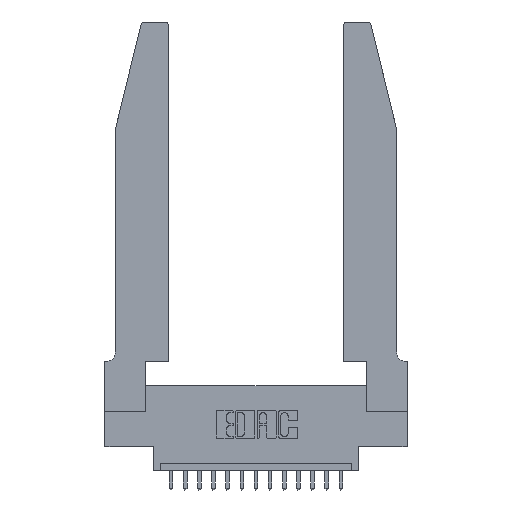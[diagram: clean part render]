
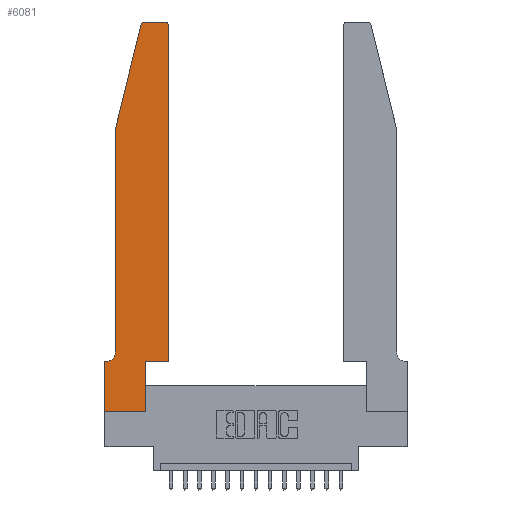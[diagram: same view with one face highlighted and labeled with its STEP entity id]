
A CAD part, top view. The second image highlights one B-rep face of the part: STEP entity #6081.
In plain terms, the highlighted planar face has unit normal (0, 0, 1).
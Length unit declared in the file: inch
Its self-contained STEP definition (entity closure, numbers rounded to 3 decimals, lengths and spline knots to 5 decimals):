
#275 = EDGE_CURVE ( 'NONE', #992, #12603, #14734, .T. ) ;
#431 = ORIENTED_EDGE ( 'NONE', *, *, #1034, .T. ) ;
#802 = LINE ( 'NONE', #11747, #1932 ) ;
#893 = ORIENTED_EDGE ( 'NONE', *, *, #7405, .T. ) ;
#992 = VERTEX_POINT ( 'NONE', #16930 ) ;
#1011 = DIRECTION ( 'NONE',  ( 1., 0., 0. ) ) ;
#1034 = EDGE_CURVE ( 'NONE', #15784, #10803, #11558, .T. ) ;
#1245 = LINE ( 'NONE', #11678, #12207 ) ;
#1253 = ORIENTED_EDGE ( 'NONE', *, *, #7828, .T. ) ;
#1406 = VECTOR ( 'NONE', #17836, 39.37008 ) ;
#1714 = VECTOR ( 'NONE', #6946, 39.37008 ) ;
#1932 = VECTOR ( 'NONE', #6489, 39.37008 ) ;
#2142 = CARTESIAN_POINT ( 'NONE',  ( 0.0755, 0.42, 0.37 ) ) ;
#2252 = ORIENTED_EDGE ( 'NONE', *, *, #5869, .T. ) ;
#2297 = ORIENTED_EDGE ( 'NONE', *, *, #18383, .T. ) ;
#2331 = EDGE_CURVE ( 'NONE', #3110, #8084, #14193, .T. ) ;
#2360 = CARTESIAN_POINT ( 'NONE',  ( 0.4505, 0.35, 0.37 ) ) ;
#2368 = LINE ( 'NONE', #11858, #17186 ) ;
#2920 = CARTESIAN_POINT ( 'NONE',  ( 0.4505, 0.35, 0.37 ) ) ;
#2996 = VECTOR ( 'NONE', #14667, 39.37008 ) ;
#3092 = EDGE_CURVE ( 'NONE', #12421, #7818, #16672, .T. ) ;
#3110 = VERTEX_POINT ( 'NONE', #2142 ) ;
#3122 = CARTESIAN_POINT ( 'NONE',  ( 0.25487, 2.72718, 0.37 ) ) ;
#3151 = DIRECTION ( 'NONE',  ( 0., -1., 0. ) ) ;
#3358 = ORIENTED_EDGE ( 'NONE', *, *, #275, .T. ) ;
#4008 = CARTESIAN_POINT ( 'NONE',  ( 0.284, 2.75, 0.37 ) ) ;
#4767 = CARTESIAN_POINT ( 'NONE',  ( 0.2865, 0., 0.37 ) ) ;
#4780 = CARTESIAN_POINT ( 'NONE',  ( 0.2605, 2.75, 0.37 ) ) ;
#5009 = CARTESIAN_POINT ( 'NONE',  ( 0.4205, 2.75, 0.37 ) ) ;
#5579 = CARTESIAN_POINT ( 'NONE',  ( 0.4505, 2.72, 0.37 ) ) ;
#5681 = LINE ( 'NONE', #9490, #6774 ) ;
#5869 = EDGE_CURVE ( 'NONE', #12247, #12972, #1245, .T. ) ;
#6023 = CARTESIAN_POINT ( 'NONE',  ( 0.4505, 0.35, 0.37 ) ) ;
#6081 = ADVANCED_FACE ( 'NONE', ( #13784 ), #17409, .T. ) ;
#6287 = EDGE_CURVE ( 'NONE', #8084, #18220, #2368, .T. ) ;
#6299 = EDGE_CURVE ( 'NONE', #10803, #992, #802, .T. ) ;
#6489 = DIRECTION ( 'NONE',  ( 0., 1., 0. ) ) ;
#6620 = ORIENTED_EDGE ( 'NONE', *, *, #6299, .T. ) ;
#6774 = VECTOR ( 'NONE', #18067, 39.37008 ) ;
#6930 = ORIENTED_EDGE ( 'NONE', *, *, #15276, .T. ) ;
#6946 = DIRECTION ( 'NONE',  ( 1., 0., 0. ) ) ;
#7000 = DIRECTION ( 'NONE',  ( 0., 0., 1. ) ) ;
#7405 = EDGE_CURVE ( 'NONE', #12603, #15984, #17155, .T. ) ;
#7805 = CARTESIAN_POINT ( 'NONE',  ( 0., 0.35, 0.37 ) ) ;
#7818 = VERTEX_POINT ( 'NONE', #4008 ) ;
#7828 = EDGE_CURVE ( 'NONE', #7818, #12247, #18034, .T. ) ;
#8000 = VECTOR ( 'NONE', #12932, 39.37008 ) ;
#8084 = VERTEX_POINT ( 'NONE', #15748 ) ;
#8209 = AXIS2_PLACEMENT_3D ( 'NONE', #16126, #17591, #13353 ) ;
#8417 = CIRCLE ( 'NONE', #18144, 0.03 ) ;
#8567 = ORIENTED_EDGE ( 'NONE', *, *, #3092, .T. ) ;
#8628 = ORIENTED_EDGE ( 'NONE', *, *, #6287, .T. ) ;
#8824 = CARTESIAN_POINT ( 'NONE',  ( 0.0755, 2., 0.37 ) ) ;
#8908 = DIRECTION ( 'NONE',  ( 0., 0., 1. ) ) ;
#9490 = CARTESIAN_POINT ( 'NONE',  ( 0., 0., 0.37 ) ) ;
#9697 = AXIS2_PLACEMENT_3D ( 'NONE', #13235, #8908, #16075 ) ;
#10175 = ORIENTED_EDGE ( 'NONE', *, *, #11659, .T. ) ;
#10605 = CARTESIAN_POINT ( 'NONE',  ( 0.0755, 2., 0.37 ) ) ;
#10803 = VERTEX_POINT ( 'NONE', #4767 ) ;
#10915 = ORIENTED_EDGE ( 'NONE', *, *, #2331, .T. ) ;
#11319 = DIRECTION ( 'NONE',  ( 1., 0., 0. ) ) ;
#11504 = DIRECTION ( 'NONE',  ( -0.239, -0.971, 0. ) ) ;
#11558 = LINE ( 'NONE', #14008, #1714 ) ;
#11659 = EDGE_CURVE ( 'NONE', #12972, #3110, #17326, .T. ) ;
#11678 = CARTESIAN_POINT ( 'NONE',  ( 0.0755, 2., 0.37 ) ) ;
#11747 = CARTESIAN_POINT ( 'NONE',  ( 0.2865, 0.35, 0.37 ) ) ;
#11858 = CARTESIAN_POINT ( 'NONE',  ( 0.0755, 0.35, 0.37 ) ) ;
#12121 = VECTOR ( 'NONE', #3151, 39.37008 ) ;
#12207 = VECTOR ( 'NONE', #11504, 39.37008 ) ;
#12247 = VERTEX_POINT ( 'NONE', #3122 ) ;
#12421 = VERTEX_POINT ( 'NONE', #5009 ) ;
#12441 = CARTESIAN_POINT ( 'NONE',  ( 0., 0., 0.37 ) ) ;
#12513 = DIRECTION ( 'NONE',  ( 0., 0., 1. ) ) ;
#12603 = VERTEX_POINT ( 'NONE', #2360 ) ;
#12932 = DIRECTION ( 'NONE',  ( 1., 0., 0. ) ) ;
#12972 = VERTEX_POINT ( 'NONE', #10605 ) ;
#12978 = EDGE_LOOP ( 'NONE', ( #8567, #1253, #2252, #10175, #10915, #8628, #2297, #431, #6620, #3358, #893, #6930 ) ) ;
#13235 = CARTESIAN_POINT ( 'NONE',  ( 0., 0.35, 0.37 ) ) ;
#13285 = DIRECTION ( 'NONE',  ( -1., 0., 0. ) ) ;
#13353 = DIRECTION ( 'NONE',  ( -1., 0., 0. ) ) ;
#13784 = FACE_OUTER_BOUND ( 'NONE', #12978, .T. ) ;
#13999 = CARTESIAN_POINT ( 'NONE',  ( 0.284, 2.72, 0.37 ) ) ;
#14008 = CARTESIAN_POINT ( 'NONE',  ( 0., 0., 0.37 ) ) ;
#14193 = CIRCLE ( 'NONE', #8209, 0.07 ) ;
#14667 = DIRECTION ( 'NONE',  ( 0., 1., 0. ) ) ;
#14734 = LINE ( 'NONE', #2920, #8000 ) ;
#15185 = CARTESIAN_POINT ( 'NONE',  ( 0.4205, 2.72, 0.37 ) ) ;
#15276 = EDGE_CURVE ( 'NONE', #15984, #12421, #8417, .T. ) ;
#15748 = CARTESIAN_POINT ( 'NONE',  ( 0.0055, 0.35, 0.37 ) ) ;
#15784 = VERTEX_POINT ( 'NONE', #12441 ) ;
#15984 = VERTEX_POINT ( 'NONE', #5579 ) ;
#16075 = DIRECTION ( 'NONE',  ( 1., 0., 0. ) ) ;
#16126 = CARTESIAN_POINT ( 'NONE',  ( 0.0055, 0.42, 0.37 ) ) ;
#16672 = LINE ( 'NONE', #4780, #1406 ) ;
#16930 = CARTESIAN_POINT ( 'NONE',  ( 0.2865, 0.35, 0.37 ) ) ;
#17155 = LINE ( 'NONE', #6023, #2996 ) ;
#17186 = VECTOR ( 'NONE', #13285, 39.37008 ) ;
#17210 = AXIS2_PLACEMENT_3D ( 'NONE', #13999, #7000, #11319 ) ;
#17326 = LINE ( 'NONE', #8824, #12121 ) ;
#17409 = PLANE ( 'NONE',  #9697 ) ;
#17591 = DIRECTION ( 'NONE',  ( 0., 0., -1. ) ) ;
#17836 = DIRECTION ( 'NONE',  ( -1., 0., 0. ) ) ;
#18034 = CIRCLE ( 'NONE', #17210, 0.03 ) ;
#18067 = DIRECTION ( 'NONE',  ( 0., -1., 0. ) ) ;
#18144 = AXIS2_PLACEMENT_3D ( 'NONE', #15185, #12513, #1011 ) ;
#18220 = VERTEX_POINT ( 'NONE', #7805 ) ;
#18383 = EDGE_CURVE ( 'NONE', #18220, #15784, #5681, .T. ) ;
